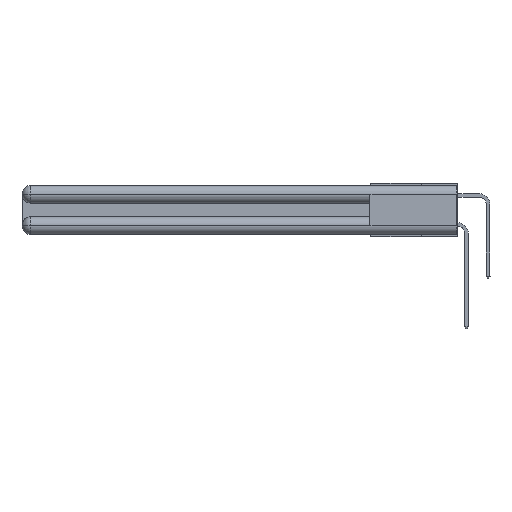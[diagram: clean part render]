
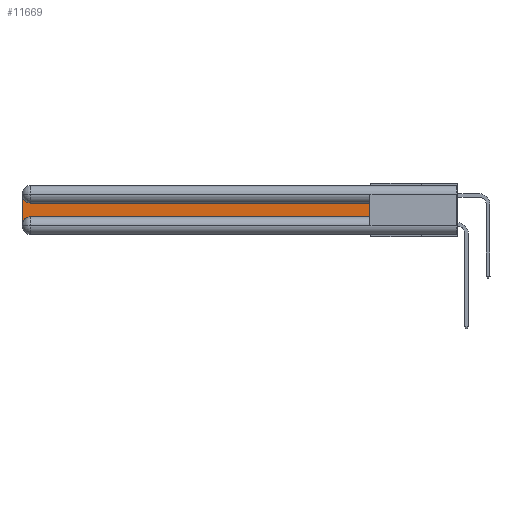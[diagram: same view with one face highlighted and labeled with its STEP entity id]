
A CAD part, left-side view. The second image highlights one B-rep face of the part: STEP entity #11669.
In plain terms, the highlighted planar face has unit normal (-1, 0, 0).
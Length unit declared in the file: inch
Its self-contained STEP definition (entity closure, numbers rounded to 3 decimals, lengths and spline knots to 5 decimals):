
#1565 = DIRECTION ( 'NONE',  ( 1., 0., 0. ) ) ;
#1652 = DIRECTION ( 'NONE',  ( 0., 0., -1. ) ) ;
#1683 = CARTESIAN_POINT ( 'NONE',  ( 0.075, 2.94, -0.2175 ) ) ;
#1718 = AXIS2_PLACEMENT_3D ( 'NONE', #13803, #11205, #18820 ) ;
#2352 = CARTESIAN_POINT ( 'NONE',  ( 0.075, 3., -0.0625 ) ) ;
#2400 = CARTESIAN_POINT ( 'NONE',  ( 0.075, 0.6, -0.1225 ) ) ;
#2748 = ORIENTED_EDGE ( 'NONE', *, *, #3394, .T. ) ;
#3055 = CARTESIAN_POINT ( 'NONE',  ( 0.075, 2.94, -0.1225 ) ) ;
#3155 = DIRECTION ( 'NONE',  ( 0., 0., -1. ) ) ;
#3361 = DIRECTION ( 'NONE',  ( 1., 0., 0. ) ) ;
#3394 = EDGE_CURVE ( 'NONE', #19979, #27558, #12545, .T. ) ;
#3464 = FACE_OUTER_BOUND ( 'NONE', #3539, .T. ) ;
#3539 = EDGE_LOOP ( 'NONE', ( #27494, #23960, #9355, #2748, #11971, #9627 ) ) ;
#5113 = VECTOR ( 'NONE', #23334, 39.37008 ) ;
#5696 = EDGE_CURVE ( 'NONE', #20132, #19979, #11142, .T. ) ;
#6786 = DIRECTION ( 'NONE',  ( 0., -1., 0. ) ) ;
#8026 = VERTEX_POINT ( 'NONE', #27678 ) ;
#9103 = CARTESIAN_POINT ( 'NONE',  ( 0.075, 2.94, -0.2775 ) ) ;
#9355 = ORIENTED_EDGE ( 'NONE', *, *, #5696, .T. ) ;
#9627 = ORIENTED_EDGE ( 'NONE', *, *, #28025, .T. ) ;
#11065 = DIRECTION ( 'NONE',  ( 0., 0., 1. ) ) ;
#11142 = LINE ( 'NONE', #30266, #14386 ) ;
#11205 = DIRECTION ( 'NONE',  ( 1., 0., 0. ) ) ;
#11669 = ADVANCED_FACE ( 'NONE', ( #3464 ), #24273, .F. ) ;
#11971 = ORIENTED_EDGE ( 'NONE', *, *, #17658, .T. ) ;
#12545 = CIRCLE ( 'NONE', #15100, 0.06 ) ;
#13803 = CARTESIAN_POINT ( 'NONE',  ( 0.075, 3., -0.1225 ) ) ;
#14386 = VECTOR ( 'NONE', #1652, 39.37008 ) ;
#14656 = VERTEX_POINT ( 'NONE', #3055 ) ;
#15100 = AXIS2_PLACEMENT_3D ( 'NONE', #9103, #1565, #32900 ) ;
#16944 = LINE ( 'NONE', #30261, #19777 ) ;
#17658 = EDGE_CURVE ( 'NONE', #27558, #20809, #16944, .T. ) ;
#18325 = EDGE_CURVE ( 'NONE', #8026, #14656, #25074, .T. ) ;
#18640 = CARTESIAN_POINT ( 'NONE',  ( 0.075, 2.94, -0.0625 ) ) ;
#18820 = DIRECTION ( 'NONE',  ( 0., 0., -1. ) ) ;
#19115 = CARTESIAN_POINT ( 'NONE',  ( 0.075, 0.6, -0.2175 ) ) ;
#19515 = EDGE_CURVE ( 'NONE', #14656, #20132, #29470, .T. ) ;
#19777 = VECTOR ( 'NONE', #6786, 39.37008 ) ;
#19979 = VERTEX_POINT ( 'NONE', #25158 ) ;
#20132 = VERTEX_POINT ( 'NONE', #2352 ) ;
#20809 = VERTEX_POINT ( 'NONE', #32613 ) ;
#23334 = DIRECTION ( 'NONE',  ( 0., 1., 0. ) ) ;
#23642 = VECTOR ( 'NONE', #11065, 39.37008 ) ;
#23960 = ORIENTED_EDGE ( 'NONE', *, *, #19515, .T. ) ;
#24273 = PLANE ( 'NONE',  #1718 ) ;
#25074 = LINE ( 'NONE', #2400, #5113 ) ;
#25158 = CARTESIAN_POINT ( 'NONE',  ( 0.075, 3., -0.2775 ) ) ;
#26115 = LINE ( 'NONE', #19115, #23642 ) ;
#27494 = ORIENTED_EDGE ( 'NONE', *, *, #18325, .T. ) ;
#27558 = VERTEX_POINT ( 'NONE', #1683 ) ;
#27678 = CARTESIAN_POINT ( 'NONE',  ( 0.075, 0.6, -0.1225 ) ) ;
#28025 = EDGE_CURVE ( 'NONE', #20809, #8026, #26115, .T. ) ;
#29470 = CIRCLE ( 'NONE', #30965, 0.06 ) ;
#30261 = CARTESIAN_POINT ( 'NONE',  ( 0.075, 0.6, -0.2175 ) ) ;
#30266 = CARTESIAN_POINT ( 'NONE',  ( 0.075, 3., -0.2175 ) ) ;
#30965 = AXIS2_PLACEMENT_3D ( 'NONE', #18640, #3361, #3155 ) ;
#32613 = CARTESIAN_POINT ( 'NONE',  ( 0.075, 0.6, -0.2175 ) ) ;
#32900 = DIRECTION ( 'NONE',  ( 0., 0., -1. ) ) ;
